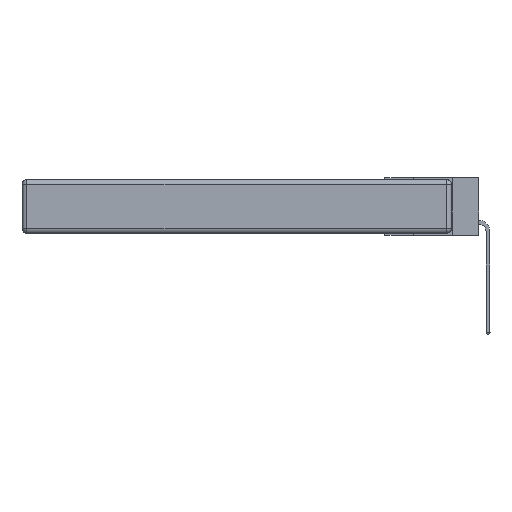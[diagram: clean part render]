
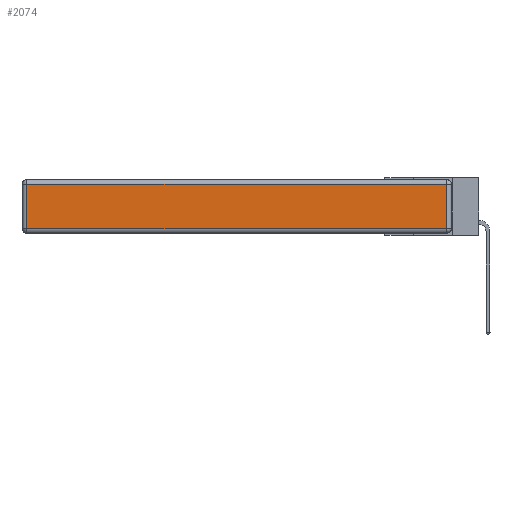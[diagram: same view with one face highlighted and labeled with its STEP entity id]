
A CAD part, left-side view. The second image highlights one B-rep face of the part: STEP entity #2074.
In plain terms, the highlighted planar face has unit normal (-1, 0, 0).
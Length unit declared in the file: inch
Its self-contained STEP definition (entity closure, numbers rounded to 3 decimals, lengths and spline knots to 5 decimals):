
#2040 = LINE ( 'NONE', #7127, #4942 ) ;
#2074 = ADVANCED_FACE ( 'NONE', ( #18144 ), #21309, .T. ) ;
#2343 = VECTOR ( 'NONE', #19829, 39.37008 ) ;
#3899 = LINE ( 'NONE', #4663, #24441 ) ;
#4663 = CARTESIAN_POINT ( 'NONE',  ( 0., 2.75, -0.03 ) ) ;
#4942 = VECTOR ( 'NONE', #5129, 39.37008 ) ;
#5129 = DIRECTION ( 'NONE',  ( 0., 0., 1. ) ) ;
#6024 = LINE ( 'NONE', #22841, #29089 ) ;
#7127 = CARTESIAN_POINT ( 'NONE',  ( 0., 0.03, -0.343 ) ) ;
#8354 = EDGE_LOOP ( 'NONE', ( #13921, #10681, #22689, #21325 ) ) ;
#8977 = DIRECTION ( 'NONE',  ( 0., 1., 0. ) ) ;
#9038 = EDGE_CURVE ( 'NONE', #14366, #28298, #3899, .T. ) ;
#10681 = ORIENTED_EDGE ( 'NONE', *, *, #23670, .T. ) ;
#12159 = DIRECTION ( 'NONE',  ( 0., 0., 1. ) ) ;
#12457 = LINE ( 'NONE', #29370, #2343 ) ;
#13921 = ORIENTED_EDGE ( 'NONE', *, *, #14157, .T. ) ;
#14157 = EDGE_CURVE ( 'NONE', #16693, #16238, #12457, .T. ) ;
#14366 = VERTEX_POINT ( 'NONE', #24931 ) ;
#16238 = VERTEX_POINT ( 'NONE', #17284 ) ;
#16693 = VERTEX_POINT ( 'NONE', #25808 ) ;
#17019 = AXIS2_PLACEMENT_3D ( 'NONE', #23628, #25924, #12159 ) ;
#17284 = CARTESIAN_POINT ( 'NONE',  ( 0., 0.03, -0.313 ) ) ;
#18144 = FACE_OUTER_BOUND ( 'NONE', #8354, .T. ) ;
#18329 = DIRECTION ( 'NONE',  ( 0., 0., -1. ) ) ;
#19210 = EDGE_CURVE ( 'NONE', #28298, #16693, #6024, .T. ) ;
#19829 = DIRECTION ( 'NONE',  ( 0., -1., 0. ) ) ;
#21309 = PLANE ( 'NONE',  #17019 ) ;
#21325 = ORIENTED_EDGE ( 'NONE', *, *, #19210, .T. ) ;
#22689 = ORIENTED_EDGE ( 'NONE', *, *, #9038, .T. ) ;
#22841 = CARTESIAN_POINT ( 'NONE',  ( 0., 2.72, -0.343 ) ) ;
#23016 = CARTESIAN_POINT ( 'NONE',  ( 0., 2.72, -0.03 ) ) ;
#23628 = CARTESIAN_POINT ( 'NONE',  ( 0., 0., -0.343 ) ) ;
#23670 = EDGE_CURVE ( 'NONE', #16238, #14366, #2040, .T. ) ;
#24441 = VECTOR ( 'NONE', #8977, 39.37008 ) ;
#24931 = CARTESIAN_POINT ( 'NONE',  ( 0., 0.03, -0.03 ) ) ;
#25808 = CARTESIAN_POINT ( 'NONE',  ( 0., 2.72, -0.313 ) ) ;
#25924 = DIRECTION ( 'NONE',  ( -1., 0., 0. ) ) ;
#28298 = VERTEX_POINT ( 'NONE', #23016 ) ;
#29089 = VECTOR ( 'NONE', #18329, 39.37008 ) ;
#29370 = CARTESIAN_POINT ( 'NONE',  ( 0., 0., -0.313 ) ) ;
